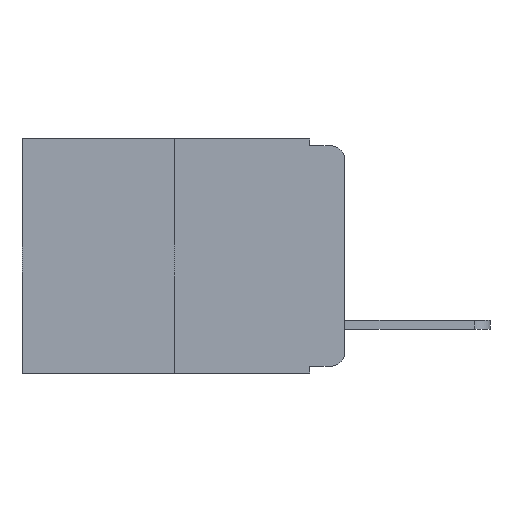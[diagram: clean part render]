
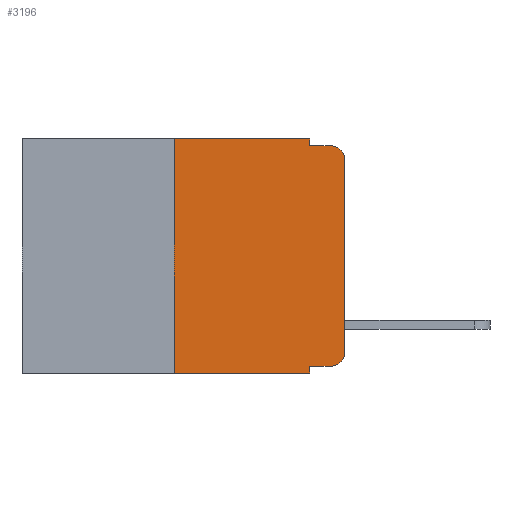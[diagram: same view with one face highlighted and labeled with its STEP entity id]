
A CAD part, left-side view. The second image highlights one B-rep face of the part: STEP entity #3196.
In plain terms, the highlighted planar face has unit normal (-1, 0, 0).
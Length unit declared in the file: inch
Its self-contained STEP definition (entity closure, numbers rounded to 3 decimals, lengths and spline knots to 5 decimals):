
#196 = LINE ( 'NONE', #7818, #10621 ) ;
#199 = ORIENTED_EDGE ( 'NONE', *, *, #5037, .F. ) ;
#300 = EDGE_CURVE ( 'NONE', #8624, #5603, #5983, .T. ) ;
#364 = ORIENTED_EDGE ( 'NONE', *, *, #300, .T. ) ;
#378 = CARTESIAN_POINT ( 'NONE',  ( 0., 0.051, -0.01 ) ) ;
#509 = EDGE_CURVE ( 'NONE', #13355, #12740, #196, .T. ) ;
#664 = ORIENTED_EDGE ( 'NONE', *, *, #509, .T. ) ;
#694 = DIRECTION ( 'NONE',  ( 0., 0., -1. ) ) ;
#787 = VERTEX_POINT ( 'NONE', #10663 ) ;
#920 = DIRECTION ( 'NONE',  ( 0., 0., 1. ) ) ;
#939 = DIRECTION ( 'NONE',  ( 0., -1., 0. ) ) ;
#1118 = DIRECTION ( 'NONE',  ( -1., 0., 0. ) ) ;
#1469 = EDGE_LOOP ( 'NONE', ( #664, #6276, #8851, #9364, #199, #11900, #364, #13322, #11594, #12220 ) ) ;
#1704 = VECTOR ( 'NONE', #920, 39.37008 ) ;
#1803 = VECTOR ( 'NONE', #9120, 39.37008 ) ;
#2048 = CARTESIAN_POINT ( 'NONE',  ( 0., 0., -0.313 ) ) ;
#2115 = LINE ( 'NONE', #12173, #12747 ) ;
#2256 = CARTESIAN_POINT ( 'NONE',  ( 0., 0.051, 0. ) ) ;
#2397 = EDGE_CURVE ( 'NONE', #12061, #7660, #4652, .T. ) ;
#2440 = VERTEX_POINT ( 'NONE', #8302 ) ;
#2687 = VECTOR ( 'NONE', #939, 39.37008 ) ;
#2717 = AXIS2_PLACEMENT_3D ( 'NONE', #7451, #1118, #8409 ) ;
#2853 = DIRECTION ( 'NONE',  ( -1., 0., 0. ) ) ;
#2867 = VECTOR ( 'NONE', #4826, 39.37008 ) ;
#3196 = ADVANCED_FACE ( 'NONE', ( #11532 ), #8998, .F. ) ;
#3243 = AXIS2_PLACEMENT_3D ( 'NONE', #10048, #7023, #694 ) ;
#3347 = CIRCLE ( 'NONE', #4535, 0.02 ) ;
#4039 = CARTESIAN_POINT ( 'NONE',  ( 0., 0.051, 0. ) ) ;
#4227 = DIRECTION ( 'NONE',  ( 0., 0., 1. ) ) ;
#4535 = AXIS2_PLACEMENT_3D ( 'NONE', #9037, #2853, #10087 ) ;
#4652 = LINE ( 'NONE', #8533, #1803 ) ;
#4676 = CARTESIAN_POINT ( 'NONE',  ( 0., 0.051, 0. ) ) ;
#4823 = CARTESIAN_POINT ( 'NONE',  ( 0., 0.473, -0.343 ) ) ;
#4826 = DIRECTION ( 'NONE',  ( 0., -1., 0. ) ) ;
#5037 = EDGE_CURVE ( 'NONE', #787, #5719, #2115, .T. ) ;
#5072 = DIRECTION ( 'NONE',  ( 0., -1., 0. ) ) ;
#5137 = CARTESIAN_POINT ( 'NONE',  ( 0., 0.051, -0.01 ) ) ;
#5149 = CARTESIAN_POINT ( 'NONE',  ( 0., 0.25, -0.343 ) ) ;
#5174 = CARTESIAN_POINT ( 'NONE',  ( 0., 0.051, -0.333 ) ) ;
#5502 = LINE ( 'NONE', #5137, #2687 ) ;
#5603 = VERTEX_POINT ( 'NONE', #10696 ) ;
#5719 = VERTEX_POINT ( 'NONE', #4676 ) ;
#5983 = LINE ( 'NONE', #4823, #2867 ) ;
#6107 = VECTOR ( 'NONE', #10171, 39.37008 ) ;
#6276 = ORIENTED_EDGE ( 'NONE', *, *, #7846, .T. ) ;
#6312 = CIRCLE ( 'NONE', #2717, 0.02 ) ;
#7023 = DIRECTION ( 'NONE',  ( 1., 0., 0. ) ) ;
#7165 = CARTESIAN_POINT ( 'NONE',  ( 0., 0.02, -0.333 ) ) ;
#7198 = VERTEX_POINT ( 'NONE', #378 ) ;
#7451 = CARTESIAN_POINT ( 'NONE',  ( 0., 0.02, -0.03 ) ) ;
#7660 = VERTEX_POINT ( 'NONE', #7165 ) ;
#7781 = EDGE_CURVE ( 'NONE', #8624, #787, #10005, .T. ) ;
#7818 = CARTESIAN_POINT ( 'NONE',  ( 0., 0., 0. ) ) ;
#7846 = EDGE_CURVE ( 'NONE', #12740, #2440, #6312, .T. ) ;
#7900 = LINE ( 'NONE', #2256, #10273 ) ;
#8302 = CARTESIAN_POINT ( 'NONE',  ( 0., 0.02, -0.01 ) ) ;
#8409 = DIRECTION ( 'NONE',  ( 0., 0., -1. ) ) ;
#8533 = CARTESIAN_POINT ( 'NONE',  ( 0., 0.051, -0.333 ) ) ;
#8624 = VERTEX_POINT ( 'NONE', #5149 ) ;
#8851 = ORIENTED_EDGE ( 'NONE', *, *, #12067, .F. ) ;
#8998 = PLANE ( 'NONE',  #3243 ) ;
#9037 = CARTESIAN_POINT ( 'NONE',  ( 0., 0.02, -0.313 ) ) ;
#9120 = DIRECTION ( 'NONE',  ( 0., -1., 0. ) ) ;
#9364 = ORIENTED_EDGE ( 'NONE', *, *, #9900, .F. ) ;
#9453 = EDGE_CURVE ( 'NONE', #12061, #5603, #7900, .T. ) ;
#9520 = DIRECTION ( 'NONE',  ( 0., 0., -1. ) ) ;
#9841 = EDGE_CURVE ( 'NONE', #7660, #13355, #3347, .T. ) ;
#9900 = EDGE_CURVE ( 'NONE', #5719, #7198, #10900, .T. ) ;
#10005 = LINE ( 'NONE', #13352, #1704 ) ;
#10048 = CARTESIAN_POINT ( 'NONE',  ( 0., 0.473, 0. ) ) ;
#10087 = DIRECTION ( 'NONE',  ( 0., 0., -1. ) ) ;
#10171 = DIRECTION ( 'NONE',  ( 0., 0., -1. ) ) ;
#10273 = VECTOR ( 'NONE', #9520, 39.37008 ) ;
#10621 = VECTOR ( 'NONE', #4227, 39.37008 ) ;
#10663 = CARTESIAN_POINT ( 'NONE',  ( 0., 0.25, 0. ) ) ;
#10696 = CARTESIAN_POINT ( 'NONE',  ( 0., 0.051, -0.343 ) ) ;
#10900 = LINE ( 'NONE', #4039, #6107 ) ;
#11532 = FACE_OUTER_BOUND ( 'NONE', #1469, .T. ) ;
#11594 = ORIENTED_EDGE ( 'NONE', *, *, #2397, .T. ) ;
#11900 = ORIENTED_EDGE ( 'NONE', *, *, #7781, .F. ) ;
#12061 = VERTEX_POINT ( 'NONE', #5174 ) ;
#12067 = EDGE_CURVE ( 'NONE', #7198, #2440, #5502, .T. ) ;
#12173 = CARTESIAN_POINT ( 'NONE',  ( 0., 0.473, 0. ) ) ;
#12220 = ORIENTED_EDGE ( 'NONE', *, *, #9841, .T. ) ;
#12740 = VERTEX_POINT ( 'NONE', #13314 ) ;
#12747 = VECTOR ( 'NONE', #5072, 39.37008 ) ;
#13314 = CARTESIAN_POINT ( 'NONE',  ( 0., 0., -0.03 ) ) ;
#13322 = ORIENTED_EDGE ( 'NONE', *, *, #9453, .F. ) ;
#13352 = CARTESIAN_POINT ( 'NONE',  ( 0., 0.25, 0. ) ) ;
#13355 = VERTEX_POINT ( 'NONE', #2048 ) ;
